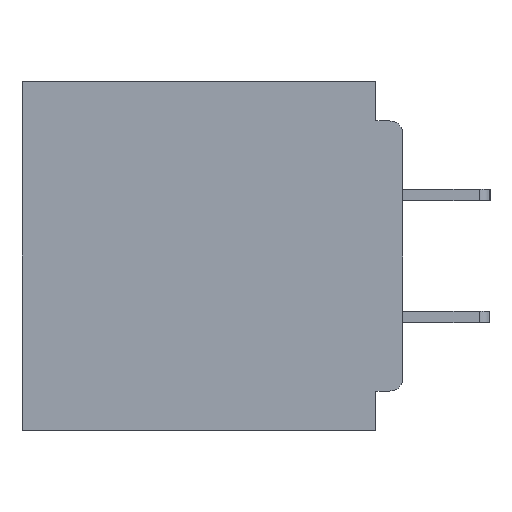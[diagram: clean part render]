
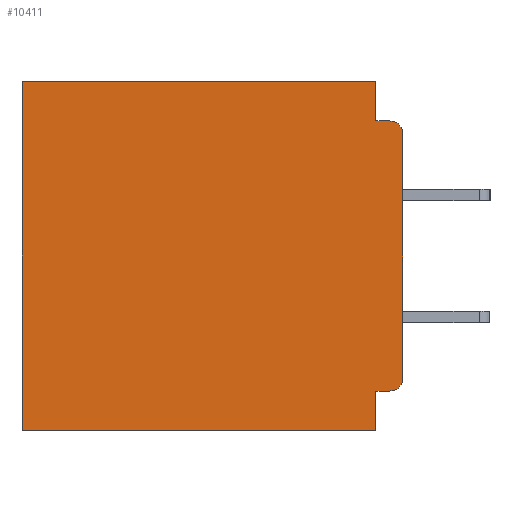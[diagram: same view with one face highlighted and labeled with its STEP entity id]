
A CAD part, left-side view. The second image highlights one B-rep face of the part: STEP entity #10411.
In plain terms, the highlighted planar face has unit normal (-1, 0, 0).
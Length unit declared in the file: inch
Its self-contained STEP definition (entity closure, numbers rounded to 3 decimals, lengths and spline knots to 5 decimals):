
#166 = VERTEX_POINT ( 'NONE', #6953 ) ;
#262 = LINE ( 'NONE', #29173, #8878 ) ;
#817 = CARTESIAN_POINT ( 'NONE',  ( 0.3, 0.015, -0.355 ) ) ;
#1914 = ORIENTED_EDGE ( 'NONE', *, *, #46417, .T. ) ;
#2757 = DIRECTION ( 'NONE',  ( 0., 1., 0. ) ) ;
#3672 = DIRECTION ( 'NONE',  ( 0., 1., 0. ) ) ;
#4167 = VERTEX_POINT ( 'NONE', #6794 ) ;
#4354 = EDGE_CURVE ( 'NONE', #41383, #34679, #262, .T. ) ;
#5372 = ORIENTED_EDGE ( 'NONE', *, *, #45936, .T. ) ;
#5816 = AXIS2_PLACEMENT_3D ( 'NONE', #39981, #18068, #43628 ) ;
#6398 = CARTESIAN_POINT ( 'NONE',  ( 0.3, 0.437, 0. ) ) ;
#6534 = ORIENTED_EDGE ( 'NONE', *, *, #15866, .F. ) ;
#6794 = CARTESIAN_POINT ( 'NONE',  ( 0.3, 0.031, -0.045 ) ) ;
#6953 = CARTESIAN_POINT ( 'NONE',  ( 0.3, 0.031, -0.355 ) ) ;
#8089 = ORIENTED_EDGE ( 'NONE', *, *, #4354, .T. ) ;
#8868 = CARTESIAN_POINT ( 'NONE',  ( 0.3, 0.031, 0. ) ) ;
#8878 = VECTOR ( 'NONE', #18480, 39.37008 ) ;
#9633 = VECTOR ( 'NONE', #16562, 39.37008 ) ;
#9677 = LINE ( 'NONE', #28582, #17101 ) ;
#9698 = EDGE_CURVE ( 'NONE', #19668, #4167, #29046, .T. ) ;
#9977 = VERTEX_POINT ( 'NONE', #21443 ) ;
#10411 = ADVANCED_FACE ( 'NONE', ( #45529 ), #34670, .F. ) ;
#10685 = VERTEX_POINT ( 'NONE', #28907 ) ;
#11293 = ORIENTED_EDGE ( 'NONE', *, *, #14258, .F. ) ;
#11728 = EDGE_CURVE ( 'NONE', #22088, #166, #41484, .T. ) ;
#12191 = VECTOR ( 'NONE', #3672, 39.37008 ) ;
#12480 = VERTEX_POINT ( 'NONE', #28441 ) ;
#13158 = LINE ( 'NONE', #20602, #32560 ) ;
#13700 = CARTESIAN_POINT ( 'NONE',  ( 0.3, 0.015, -0.34 ) ) ;
#14258 = EDGE_CURVE ( 'NONE', #10685, #12480, #13158, .T. ) ;
#15752 = ORIENTED_EDGE ( 'NONE', *, *, #9698, .F. ) ;
#15866 = EDGE_CURVE ( 'NONE', #4167, #46641, #9677, .T. ) ;
#16305 = EDGE_CURVE ( 'NONE', #166, #9977, #27910, .T. ) ;
#16471 = DIRECTION ( 'NONE',  ( 1., 0., 0. ) ) ;
#16562 = DIRECTION ( 'NONE',  ( 0., 0., -1. ) ) ;
#17101 = VECTOR ( 'NONE', #21381, 39.37008 ) ;
#17246 = CARTESIAN_POINT ( 'NONE',  ( 0.3, 0., 0. ) ) ;
#17389 = DIRECTION ( 'NONE',  ( 0., 0., -1. ) ) ;
#18068 = DIRECTION ( 'NONE',  ( -1., 0., 0. ) ) ;
#18480 = DIRECTION ( 'NONE',  ( 0., 0., -1. ) ) ;
#18488 = CARTESIAN_POINT ( 'NONE',  ( 0.3, 0.437, -0.4 ) ) ;
#19668 = VERTEX_POINT ( 'NONE', #24423 ) ;
#19694 = EDGE_CURVE ( 'NONE', #19668, #41383, #40751, .T. ) ;
#20602 = CARTESIAN_POINT ( 'NONE',  ( 0.3, 0., -0.4 ) ) ;
#20880 = DIRECTION ( 'NONE',  ( 0., 1., 0. ) ) ;
#21265 = VECTOR ( 'NONE', #20880, 39.37008 ) ;
#21381 = DIRECTION ( 'NONE',  ( 0., -1., 0. ) ) ;
#21443 = CARTESIAN_POINT ( 'NONE',  ( 0.3, 0.031, -0.4 ) ) ;
#22088 = VERTEX_POINT ( 'NONE', #817 ) ;
#22461 = EDGE_LOOP ( 'NONE', ( #11293, #5372, #6534, #15752, #32674, #8089, #45682, #32622, #35621, #1914 ) ) ;
#24293 = DIRECTION ( 'NONE',  ( 0., 0., -1. ) ) ;
#24423 = CARTESIAN_POINT ( 'NONE',  ( 0.3, 0.031, 0. ) ) ;
#24831 = CARTESIAN_POINT ( 'NONE',  ( 0.3, 0., -0.355 ) ) ;
#24842 = VECTOR ( 'NONE', #2757, 39.37008 ) ;
#27074 = DIRECTION ( 'NONE',  ( 0., 0., -1. ) ) ;
#27344 = CARTESIAN_POINT ( 'NONE',  ( 0.3, 0., -0.4 ) ) ;
#27900 = VECTOR ( 'NONE', #27074, 39.37008 ) ;
#27910 = LINE ( 'NONE', #45761, #9633 ) ;
#28441 = CARTESIAN_POINT ( 'NONE',  ( 0.3, 0., -0.34 ) ) ;
#28582 = CARTESIAN_POINT ( 'NONE',  ( 0.3, 0., -0.045 ) ) ;
#28907 = CARTESIAN_POINT ( 'NONE',  ( 0.3, 0., -0.06 ) ) ;
#29046 = LINE ( 'NONE', #8868, #27900 ) ;
#29115 = CIRCLE ( 'NONE', #5816, 0.015 ) ;
#29173 = CARTESIAN_POINT ( 'NONE',  ( 0.3, 0.437, -0.4 ) ) ;
#31659 = AXIS2_PLACEMENT_3D ( 'NONE', #27344, #16471, #42074 ) ;
#32560 = VECTOR ( 'NONE', #24293, 39.37008 ) ;
#32622 = ORIENTED_EDGE ( 'NONE', *, *, #16305, .F. ) ;
#32674 = ORIENTED_EDGE ( 'NONE', *, *, #19694, .T. ) ;
#34670 = PLANE ( 'NONE',  #31659 ) ;
#34679 = VERTEX_POINT ( 'NONE', #18488 ) ;
#35621 = ORIENTED_EDGE ( 'NONE', *, *, #11728, .F. ) ;
#39299 = DIRECTION ( 'NONE',  ( -1., 0., 0. ) ) ;
#39981 = CARTESIAN_POINT ( 'NONE',  ( 0.3, 0.015, -0.06 ) ) ;
#40385 = CARTESIAN_POINT ( 'NONE',  ( 0.3, 0.015, -0.045 ) ) ;
#40751 = LINE ( 'NONE', #17246, #21265 ) ;
#41383 = VERTEX_POINT ( 'NONE', #6398 ) ;
#41388 = LINE ( 'NONE', #43805, #12191 ) ;
#41484 = LINE ( 'NONE', #24831, #24842 ) ;
#42074 = DIRECTION ( 'NONE',  ( 0., 0., -1. ) ) ;
#43454 = EDGE_CURVE ( 'NONE', #9977, #34679, #41388, .T. ) ;
#43628 = DIRECTION ( 'NONE',  ( 0., 0., -1. ) ) ;
#43805 = CARTESIAN_POINT ( 'NONE',  ( 0.3, 0., -0.4 ) ) ;
#44142 = AXIS2_PLACEMENT_3D ( 'NONE', #13700, #39299, #17389 ) ;
#45529 = FACE_OUTER_BOUND ( 'NONE', #22461, .T. ) ;
#45682 = ORIENTED_EDGE ( 'NONE', *, *, #43454, .F. ) ;
#45761 = CARTESIAN_POINT ( 'NONE',  ( 0.3, 0.031, -0.4 ) ) ;
#45936 = EDGE_CURVE ( 'NONE', #10685, #46641, #29115, .T. ) ;
#46170 = CIRCLE ( 'NONE', #44142, 0.015 ) ;
#46417 = EDGE_CURVE ( 'NONE', #22088, #12480, #46170, .T. ) ;
#46641 = VERTEX_POINT ( 'NONE', #40385 ) ;
